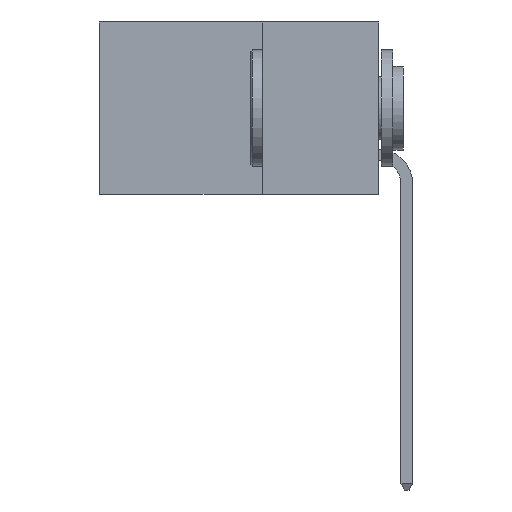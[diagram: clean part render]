
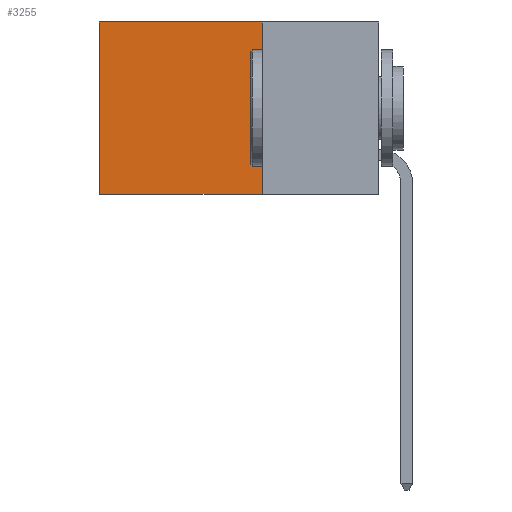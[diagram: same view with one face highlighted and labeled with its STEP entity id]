
A CAD part, left-side view. The second image highlights one B-rep face of the part: STEP entity #3255.
In plain terms, the highlighted planar face has unit normal (-1, 0, 0).
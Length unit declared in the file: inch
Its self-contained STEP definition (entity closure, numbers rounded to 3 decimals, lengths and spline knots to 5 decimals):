
#100 = VECTOR ( 'NONE', #11094, 39.37008 ) ;
#300 = ORIENTED_EDGE ( 'NONE', *, *, #8940, .F. ) ;
#358 = AXIS2_PLACEMENT_3D ( 'NONE', #6037, #5748, #5764 ) ;
#1001 = CARTESIAN_POINT ( 'NONE',  ( 0.2615, 0.25, -0.37 ) ) ;
#1346 = LINE ( 'NONE', #7879, #11818 ) ;
#2120 = EDGE_CURVE ( 'NONE', #17027, #13689, #14962, .T. ) ;
#3107 = CARTESIAN_POINT ( 'NONE',  ( 0.2615, 0.6, 0. ) ) ;
#3255 = ADVANCED_FACE ( 'NONE', ( #15563 ), #7852, .F. ) ;
#3602 = ORIENTED_EDGE ( 'NONE', *, *, #17220, .T. ) ;
#3744 = ORIENTED_EDGE ( 'NONE', *, *, #7290, .T. ) ;
#4329 = LINE ( 'NONE', #12621, #15112 ) ;
#5748 = DIRECTION ( 'NONE',  ( 1., 0., 0. ) ) ;
#5764 = DIRECTION ( 'NONE',  ( 0., 0., -1. ) ) ;
#6037 = CARTESIAN_POINT ( 'NONE',  ( 0.2615, 0.25, -0.37 ) ) ;
#7290 = EDGE_CURVE ( 'NONE', #7709, #12941, #7362, .T. ) ;
#7362 = LINE ( 'NONE', #11270, #100 ) ;
#7709 = VERTEX_POINT ( 'NONE', #3107 ) ;
#7852 = PLANE ( 'NONE',  #358 ) ;
#7879 = CARTESIAN_POINT ( 'NONE',  ( 0.2615, 0.25, 0. ) ) ;
#8940 = EDGE_CURVE ( 'NONE', #13689, #12941, #4329, .T. ) ;
#10547 = CARTESIAN_POINT ( 'NONE',  ( 0.2615, 0.6, -0.37 ) ) ;
#11094 = DIRECTION ( 'NONE',  ( 0., 0., -1. ) ) ;
#11270 = CARTESIAN_POINT ( 'NONE',  ( 0.2615, 0.6, -0.37 ) ) ;
#11584 = CARTESIAN_POINT ( 'NONE',  ( 0.2615, 0.25, 0. ) ) ;
#11818 = VECTOR ( 'NONE', #16218, 39.37008 ) ;
#12181 = DIRECTION ( 'NONE',  ( 0., 1., 0. ) ) ;
#12621 = CARTESIAN_POINT ( 'NONE',  ( 0.2615, 0.25, -0.37 ) ) ;
#12641 = EDGE_LOOP ( 'NONE', ( #3744, #300, #13920, #3602 ) ) ;
#12941 = VERTEX_POINT ( 'NONE', #10547 ) ;
#13689 = VERTEX_POINT ( 'NONE', #1001 ) ;
#13920 = ORIENTED_EDGE ( 'NONE', *, *, #2120, .F. ) ;
#14962 = LINE ( 'NONE', #15092, #15396 ) ;
#15092 = CARTESIAN_POINT ( 'NONE',  ( 0.2615, 0.25, -0.37 ) ) ;
#15112 = VECTOR ( 'NONE', #12181, 39.37008 ) ;
#15396 = VECTOR ( 'NONE', #17136, 39.37008 ) ;
#15563 = FACE_OUTER_BOUND ( 'NONE', #12641, .T. ) ;
#16218 = DIRECTION ( 'NONE',  ( 0., 1., 0. ) ) ;
#17027 = VERTEX_POINT ( 'NONE', #11584 ) ;
#17136 = DIRECTION ( 'NONE',  ( 0., 0., -1. ) ) ;
#17220 = EDGE_CURVE ( 'NONE', #17027, #7709, #1346, .T. ) ;
